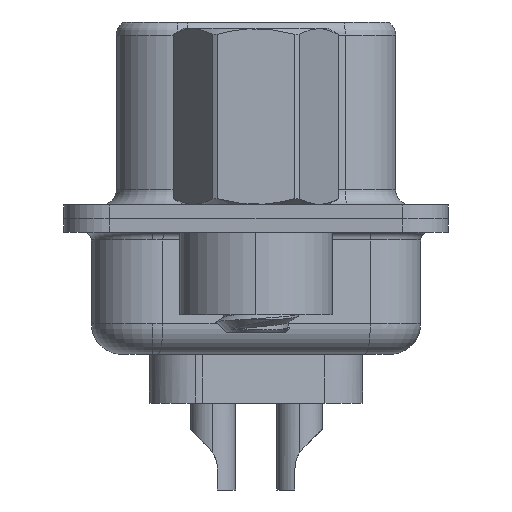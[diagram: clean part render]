
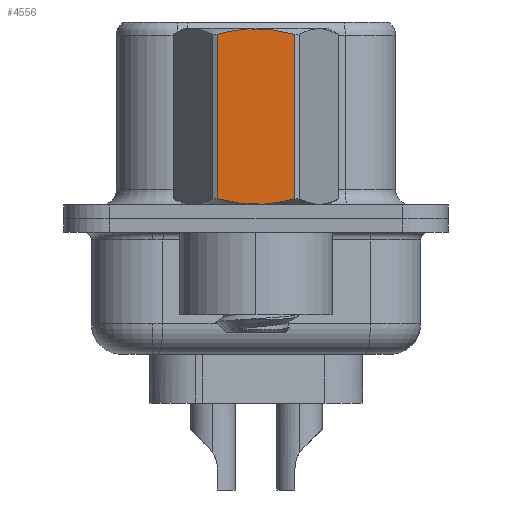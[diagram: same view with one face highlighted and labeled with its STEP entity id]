
A CAD part, left-side view. The second image highlights one B-rep face of the part: STEP entity #4556.
In plain terms, the highlighted planar face has unit normal (-1, 0, 0).
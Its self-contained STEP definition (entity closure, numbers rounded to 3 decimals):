
#1049 = CARTESIAN_POINT ( 'NONE',  ( -2.381, -1.273, 6.048 ) ) ;
#1130 = CARTESIAN_POINT ( 'NONE',  ( -2.381, 1.065, 6.104 ) ) ;
#1450 = CARTESIAN_POINT ( 'NONE',  ( -2.381, -0.432, 0.485 ) ) ;
#1840 = CARTESIAN_POINT ( 'NONE',  ( -2.381, -1.273, 0.652 ) ) ;
#2697 = VERTEX_POINT ( 'NONE', #22853 ) ;
#2996 = DIRECTION ( 'NONE',  ( 0., -1., 0. ) ) ;
#3156 = AXIS2_PLACEMENT_3D ( 'NONE', #11974, #10819, #2996 ) ;
#3364 = CARTESIAN_POINT ( 'NONE',  ( -2.381, -1.066, 0.596 ) ) ;
#4157 = ORIENTED_EDGE ( 'NONE', *, *, #17121, .T. ) ;
#4556 = ADVANCED_FACE ( 'NONE', ( #11747 ), #15096, .T. ) ;
#5935 = B_SPLINE_CURVE_WITH_KNOTS ( 'NONE', 3,
 ( #17850, #19570, #21533, #10746, #23339, #12582, #1450, #14391, #3364, #16192 ),
 .UNSPECIFIED., .F., .F.,
 ( 4, 2, 2, 2, 4 ),
 ( 0.003, 0.003, 0.004, 0.004, 0.005 ),
 .UNSPECIFIED. ) ;
#6761 = CARTESIAN_POINT ( 'NONE',  ( -2.381, -1.273, 3.792 ) ) ;
#8146 = VERTEX_POINT ( 'NONE', #1840 ) ;
#8545 = VECTOR ( 'NONE', #9896, 1000. ) ;
#8592 = CARTESIAN_POINT ( 'NONE',  ( -2.381, -0.432, 6.215 ) ) ;
#8966 = EDGE_CURVE ( 'NONE', #19337, #8146, #5935, .T. ) ;
#9896 = DIRECTION ( 'NONE',  ( 0., 0., -1. ) ) ;
#9954 = EDGE_CURVE ( 'NONE', #2697, #19337, #17597, .T. ) ;
#10430 = CARTESIAN_POINT ( 'NONE',  ( -2.381, 0.215, 6.232 ) ) ;
#10578 = LINE ( 'NONE', #6761, #14831 ) ;
#10746 = CARTESIAN_POINT ( 'NONE',  ( -2.381, 0.428, 0.485 ) ) ;
#10819 = DIRECTION ( 'NONE',  ( -1., 0., 0. ) ) ;
#11747 = FACE_OUTER_BOUND ( 'NONE', #19809, .T. ) ;
#11974 = CARTESIAN_POINT ( 'NONE',  ( -2.381, 1.375, -3.75 ) ) ;
#12278 = CARTESIAN_POINT ( 'NONE',  ( -2.381, 0.853, 6.151 ) ) ;
#12404 = ORIENTED_EDGE ( 'NONE', *, *, #9954, .T. ) ;
#12582 = CARTESIAN_POINT ( 'NONE',  ( -2.381, -0.215, 0.468 ) ) ;
#14088 = CARTESIAN_POINT ( 'NONE',  ( -2.381, 1.273, 6.048 ) ) ;
#14391 = CARTESIAN_POINT ( 'NONE',  ( -2.381, -0.858, 0.55 ) ) ;
#14831 = VECTOR ( 'NONE', #17573, 1000. ) ;
#15096 = PLANE ( 'NONE',  #3156 ) ;
#16192 = CARTESIAN_POINT ( 'NONE',  ( -2.381, -1.273, 0.652 ) ) ;
#16279 = CARTESIAN_POINT ( 'NONE',  ( -2.381, -1.273, 6.048 ) ) ;
#17121 = EDGE_CURVE ( 'NONE', #19334, #2697, #18107, .T. ) ;
#17573 = DIRECTION ( 'NONE',  ( 0., 0., 1. ) ) ;
#17597 = LINE ( 'NONE', #22510, #8545 ) ;
#17818 = EDGE_CURVE ( 'NONE', #8146, #19334, #10578, .T. ) ;
#17850 = CARTESIAN_POINT ( 'NONE',  ( -2.381, 1.273, 0.652 ) ) ;
#18107 = B_SPLINE_CURVE_WITH_KNOTS ( 'NONE', 3,
 ( #1049, #22962, #19407, #8592, #21211, #10430, #23034, #12278, #1130, #14088 ),
 .UNSPECIFIED., .F., .F.,
 ( 4, 2, 2, 2, 4 ),
 ( 0.001, 0.002, 0.002, 0.003, 0.004 ),
 .UNSPECIFIED. ) ;
#18193 = ORIENTED_EDGE ( 'NONE', *, *, #17818, .T. ) ;
#19039 = ORIENTED_EDGE ( 'NONE', *, *, #8966, .T. ) ;
#19334 = VERTEX_POINT ( 'NONE', #16279 ) ;
#19337 = VERTEX_POINT ( 'NONE', #20358 ) ;
#19407 = CARTESIAN_POINT ( 'NONE',  ( -2.381, -0.858, 6.15 ) ) ;
#19570 = CARTESIAN_POINT ( 'NONE',  ( -2.381, 1.065, 0.596 ) ) ;
#19809 = EDGE_LOOP ( 'NONE', ( #19039, #18193, #4157, #12404 ) ) ;
#20358 = CARTESIAN_POINT ( 'NONE',  ( -2.381, 1.273, 0.652 ) ) ;
#21211 = CARTESIAN_POINT ( 'NONE',  ( -2.381, -0.215, 6.232 ) ) ;
#21533 = CARTESIAN_POINT ( 'NONE',  ( -2.381, 0.853, 0.549 ) ) ;
#22510 = CARTESIAN_POINT ( 'NONE',  ( -2.381, 1.273, 3.792 ) ) ;
#22853 = CARTESIAN_POINT ( 'NONE',  ( -2.381, 1.273, 6.048 ) ) ;
#22962 = CARTESIAN_POINT ( 'NONE',  ( -2.381, -1.066, 6.104 ) ) ;
#23034 = CARTESIAN_POINT ( 'NONE',  ( -2.381, 0.428, 6.215 ) ) ;
#23339 = CARTESIAN_POINT ( 'NONE',  ( -2.381, 0.215, 0.468 ) ) ;
